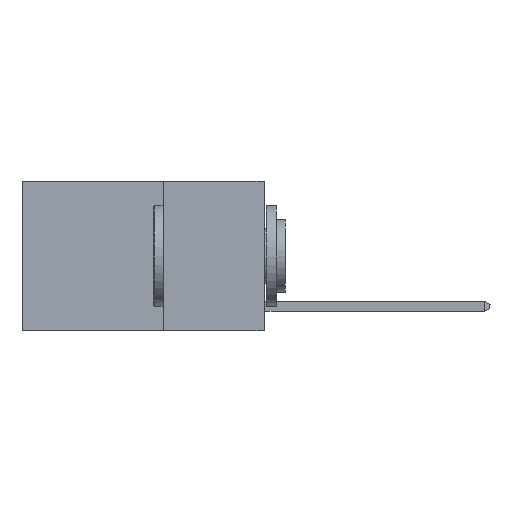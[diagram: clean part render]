
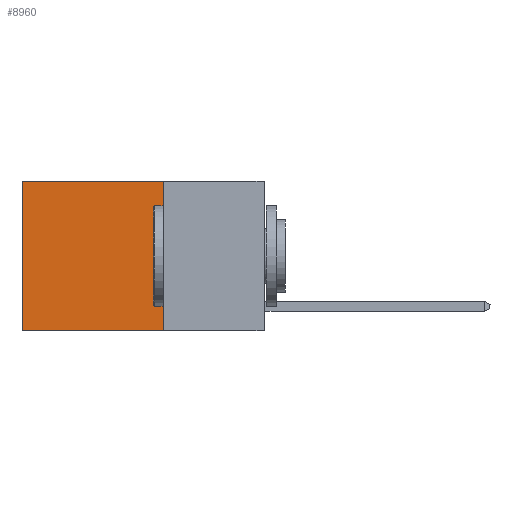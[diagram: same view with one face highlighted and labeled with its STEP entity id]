
A CAD part, left-side view. The second image highlights one B-rep face of the part: STEP entity #8960.
In plain terms, the highlighted planar face has unit normal (-1, 0, 0).
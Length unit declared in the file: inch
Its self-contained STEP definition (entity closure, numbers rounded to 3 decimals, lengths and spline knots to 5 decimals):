
#217 = AXIS2_PLACEMENT_3D ( 'NONE', #2826, #11571, #5025 ) ;
#574 = LINE ( 'NONE', #6448, #6440 ) ;
#614 = VERTEX_POINT ( 'NONE', #10332 ) ;
#780 = DIRECTION ( 'NONE',  ( 0., 0., -1. ) ) ;
#1399 = VERTEX_POINT ( 'NONE', #6382 ) ;
#1636 = ORIENTED_EDGE ( 'NONE', *, *, #2216, .F. ) ;
#1713 = PLANE ( 'NONE',  #217 ) ;
#2216 = EDGE_CURVE ( 'NONE', #1399, #614, #574, .T. ) ;
#2826 = CARTESIAN_POINT ( 'NONE',  ( 0.2625, 0.25, 0. ) ) ;
#2902 = CARTESIAN_POINT ( 'NONE',  ( 0.2625, 0.25, 0. ) ) ;
#2903 = VERTEX_POINT ( 'NONE', #3045 ) ;
#2920 = LINE ( 'NONE', #2902, #11290 ) ;
#3045 = CARTESIAN_POINT ( 'NONE',  ( 0.2625, 0.25, 0. ) ) ;
#3444 = VERTEX_POINT ( 'NONE', #9207 ) ;
#3504 = VECTOR ( 'NONE', #12611, 39.37008 ) ;
#4216 = LINE ( 'NONE', #5135, #9773 ) ;
#5025 = DIRECTION ( 'NONE',  ( 0., 0., -1. ) ) ;
#5135 = CARTESIAN_POINT ( 'NONE',  ( 0.2625, 0.25, 0. ) ) ;
#5550 = EDGE_CURVE ( 'NONE', #2903, #3444, #2920, .T. ) ;
#6205 = DIRECTION ( 'NONE',  ( 0., 1., 0. ) ) ;
#6382 = CARTESIAN_POINT ( 'NONE',  ( 0.2625, 0.25, -0.37 ) ) ;
#6440 = VECTOR ( 'NONE', #6205, 39.37008 ) ;
#6448 = CARTESIAN_POINT ( 'NONE',  ( 0.2625, 0.25, -0.37 ) ) ;
#6474 = LINE ( 'NONE', #7181, #3504 ) ;
#6853 = ORIENTED_EDGE ( 'NONE', *, *, #5550, .T. ) ;
#7181 = CARTESIAN_POINT ( 'NONE',  ( 0.2625, 0.6, 0. ) ) ;
#8320 = EDGE_CURVE ( 'NONE', #2903, #1399, #4216, .T. ) ;
#8502 = DIRECTION ( 'NONE',  ( 0., 1., 0. ) ) ;
#8960 = ADVANCED_FACE ( 'NONE', ( #12756 ), #1713, .F. ) ;
#9207 = CARTESIAN_POINT ( 'NONE',  ( 0.2625, 0.6, 0. ) ) ;
#9512 = EDGE_CURVE ( 'NONE', #3444, #614, #6474, .T. ) ;
#9773 = VECTOR ( 'NONE', #780, 39.37008 ) ;
#10332 = CARTESIAN_POINT ( 'NONE',  ( 0.2625, 0.6, -0.37 ) ) ;
#11290 = VECTOR ( 'NONE', #8502, 39.37008 ) ;
#11571 = DIRECTION ( 'NONE',  ( 1., 0., 0. ) ) ;
#11911 = EDGE_LOOP ( 'NONE', ( #13116, #1636, #13320, #6853 ) ) ;
#12611 = DIRECTION ( 'NONE',  ( 0., 0., -1. ) ) ;
#12756 = FACE_OUTER_BOUND ( 'NONE', #11911, .T. ) ;
#13116 = ORIENTED_EDGE ( 'NONE', *, *, #9512, .T. ) ;
#13320 = ORIENTED_EDGE ( 'NONE', *, *, #8320, .F. ) ;
